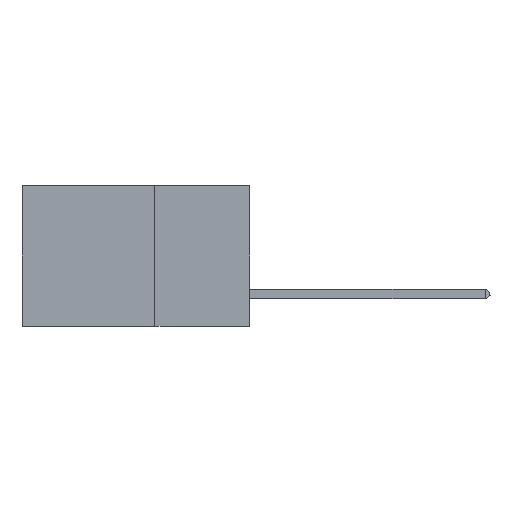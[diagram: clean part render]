
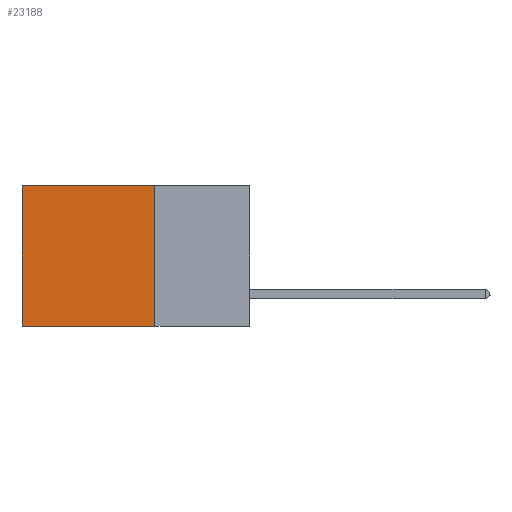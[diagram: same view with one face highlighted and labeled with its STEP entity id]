
A CAD part, left-side view. The second image highlights one B-rep face of the part: STEP entity #23188.
In plain terms, the highlighted planar face has unit normal (-1, 0, 0).
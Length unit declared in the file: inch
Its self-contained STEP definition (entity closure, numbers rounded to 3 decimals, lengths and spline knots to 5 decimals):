
#998 = CARTESIAN_POINT ( 'NONE',  ( 0.2875, 0.25, 0. ) ) ;
#1104 = FACE_OUTER_BOUND ( 'NONE', #4593, .T. ) ;
#1665 = CARTESIAN_POINT ( 'NONE',  ( 0.2875, 0.25, 0. ) ) ;
#2776 = CARTESIAN_POINT ( 'NONE',  ( 0.2875, 0.25, 0. ) ) ;
#3078 = LINE ( 'NONE', #22407, #19338 ) ;
#4071 = DIRECTION ( 'NONE',  ( 1., 0., 0. ) ) ;
#4580 = VERTEX_POINT ( 'NONE', #16471 ) ;
#4593 = EDGE_LOOP ( 'NONE', ( #24055, #10003, #24655, #22910 ) ) ;
#5852 = LINE ( 'NONE', #1665, #9222 ) ;
#6010 = DIRECTION ( 'NONE',  ( 0., 1., 0. ) ) ;
#6043 = CARTESIAN_POINT ( 'NONE',  ( 0.2875, 0.25, 0. ) ) ;
#6538 = LINE ( 'NONE', #2776, #7465 ) ;
#7465 = VECTOR ( 'NONE', #8869, 39.37008 ) ;
#8589 = DIRECTION ( 'NONE',  ( 0., 0., -1. ) ) ;
#8869 = DIRECTION ( 'NONE',  ( 0., 1., 0. ) ) ;
#8913 = CARTESIAN_POINT ( 'NONE',  ( 0.2875, 0.6, -0.37 ) ) ;
#9222 = VECTOR ( 'NONE', #15432, 39.37008 ) ;
#9692 = VECTOR ( 'NONE', #6010, 39.37008 ) ;
#10003 = ORIENTED_EDGE ( 'NONE', *, *, #23818, .F. ) ;
#10171 = PLANE ( 'NONE',  #23079 ) ;
#10406 = EDGE_CURVE ( 'NONE', #11672, #4580, #6538, .T. ) ;
#11074 = VERTEX_POINT ( 'NONE', #24640 ) ;
#11672 = VERTEX_POINT ( 'NONE', #998 ) ;
#12824 = EDGE_CURVE ( 'NONE', #4580, #24140, #3078, .T. ) ;
#14163 = CARTESIAN_POINT ( 'NONE',  ( 0.2875, 0.25, -0.37 ) ) ;
#15432 = DIRECTION ( 'NONE',  ( 0., 0., -1. ) ) ;
#16471 = CARTESIAN_POINT ( 'NONE',  ( 0.2875, 0.6, 0. ) ) ;
#19338 = VECTOR ( 'NONE', #8589, 39.37008 ) ;
#19845 = DIRECTION ( 'NONE',  ( 0., 0., -1. ) ) ;
#21634 = LINE ( 'NONE', #14163, #9692 ) ;
#22407 = CARTESIAN_POINT ( 'NONE',  ( 0.2875, 0.6, 0. ) ) ;
#22910 = ORIENTED_EDGE ( 'NONE', *, *, #10406, .T. ) ;
#23079 = AXIS2_PLACEMENT_3D ( 'NONE', #6043, #4071, #19845 ) ;
#23188 = ADVANCED_FACE ( 'NONE', ( #1104 ), #10171, .F. ) ;
#23818 = EDGE_CURVE ( 'NONE', #11074, #24140, #21634, .T. ) ;
#24055 = ORIENTED_EDGE ( 'NONE', *, *, #12824, .T. ) ;
#24140 = VERTEX_POINT ( 'NONE', #8913 ) ;
#24640 = CARTESIAN_POINT ( 'NONE',  ( 0.2875, 0.25, -0.37 ) ) ;
#24655 = ORIENTED_EDGE ( 'NONE', *, *, #24997, .F. ) ;
#24997 = EDGE_CURVE ( 'NONE', #11672, #11074, #5852, .T. ) ;
